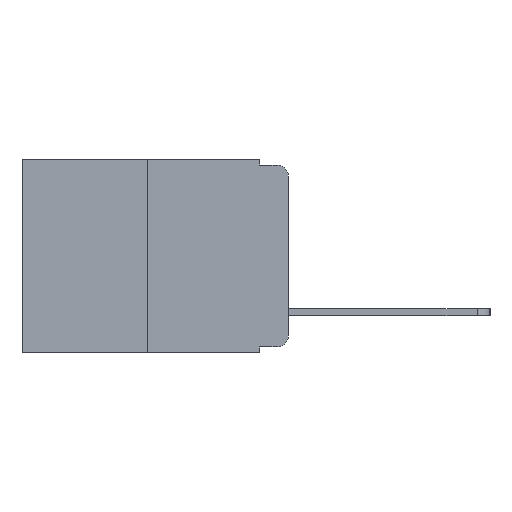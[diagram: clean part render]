
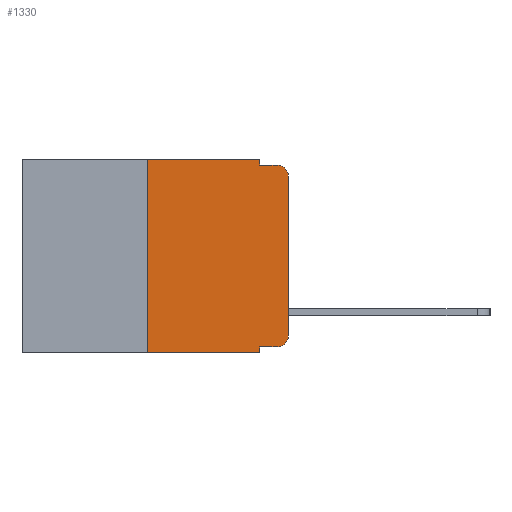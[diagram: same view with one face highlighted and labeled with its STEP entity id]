
A CAD part, left-side view. The second image highlights one B-rep face of the part: STEP entity #1330.
In plain terms, the highlighted planar face has unit normal (-1, 0, 0).
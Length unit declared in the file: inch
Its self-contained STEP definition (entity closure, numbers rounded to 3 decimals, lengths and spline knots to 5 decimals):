
#239 = CARTESIAN_POINT ( 'NONE',  ( 0., 0.473, 0. ) ) ;
#452 = CARTESIAN_POINT ( 'NONE',  ( 0., 0.25, 0. ) ) ;
#518 = DIRECTION ( 'NONE',  ( 0., -1., 0. ) ) ;
#803 = DIRECTION ( 'NONE',  ( 0., 0., 1. ) ) ;
#1142 = CARTESIAN_POINT ( 'NONE',  ( 0., 0.051, -0.01 ) ) ;
#1220 = VERTEX_POINT ( 'NONE', #11399 ) ;
#1290 = LINE ( 'NONE', #6276, #6802 ) ;
#1330 = ADVANCED_FACE ( 'NONE', ( #11483 ), #2594, .F. ) ;
#1460 = LINE ( 'NONE', #11569, #6978 ) ;
#1478 = DIRECTION ( 'NONE',  ( 0., 0., -1. ) ) ;
#1494 = DIRECTION ( 'NONE',  ( 0., -1., 0. ) ) ;
#1685 = DIRECTION ( 'NONE',  ( 0., 0., 1. ) ) ;
#1950 = DIRECTION ( 'NONE',  ( 0., 0., -1. ) ) ;
#2337 = CARTESIAN_POINT ( 'NONE',  ( 0., 0.051, 0. ) ) ;
#2455 = DIRECTION ( 'NONE',  ( 0., 0., -1. ) ) ;
#2460 = VERTEX_POINT ( 'NONE', #4876 ) ;
#2469 = DIRECTION ( 'NONE',  ( 1., 0., 0. ) ) ;
#2594 = PLANE ( 'NONE',  #12680 ) ;
#2900 = CARTESIAN_POINT ( 'NONE',  ( 0., 0.051, -0.01 ) ) ;
#2951 = CIRCLE ( 'NONE', #4506, 0.02 ) ;
#3138 = LINE ( 'NONE', #9721, #13435 ) ;
#3507 = CARTESIAN_POINT ( 'NONE',  ( 0., 0.02, -0.03 ) ) ;
#3771 = VERTEX_POINT ( 'NONE', #1142 ) ;
#4267 = CARTESIAN_POINT ( 'NONE',  ( 0., 0.02, -0.01 ) ) ;
#4317 = LINE ( 'NONE', #452, #6787 ) ;
#4451 = CARTESIAN_POINT ( 'NONE',  ( 0., 0., -0.03 ) ) ;
#4480 = LINE ( 'NONE', #13424, #9572 ) ;
#4506 = AXIS2_PLACEMENT_3D ( 'NONE', #11437, #5471, #12399 ) ;
#4597 = DIRECTION ( 'NONE',  ( 0., 0., -1. ) ) ;
#4876 = CARTESIAN_POINT ( 'NONE',  ( 0., 0.02, -0.333 ) ) ;
#5471 = DIRECTION ( 'NONE',  ( -1., 0., 0. ) ) ;
#5901 = CARTESIAN_POINT ( 'NONE',  ( 0., 0.25, -0.343 ) ) ;
#6015 = EDGE_LOOP ( 'NONE', ( #7263, #7251, #7418, #7274, #7289, #7098, #7149, #6641, #9704, #9143 ) ) ;
#6092 = VERTEX_POINT ( 'NONE', #10795 ) ;
#6276 = CARTESIAN_POINT ( 'NONE',  ( 0., 0., 0. ) ) ;
#6279 = EDGE_CURVE ( 'NONE', #3771, #13244, #11553, .T. ) ;
#6436 = EDGE_CURVE ( 'NONE', #8540, #11033, #1290, .T. ) ;
#6577 = EDGE_CURVE ( 'NONE', #2460, #8540, #2951, .T. ) ;
#6641 = ORIENTED_EDGE ( 'NONE', *, *, #6742, .F. ) ;
#6650 = EDGE_CURVE ( 'NONE', #1220, #2460, #1460, .T. ) ;
#6742 = EDGE_CURVE ( 'NONE', #1220, #9616, #3138, .T. ) ;
#6758 = LINE ( 'NONE', #239, #11659 ) ;
#6787 = VECTOR ( 'NONE', #1685, 39.37008 ) ;
#6802 = VECTOR ( 'NONE', #803, 39.37008 ) ;
#6820 = EDGE_CURVE ( 'NONE', #8948, #6092, #4317, .T. ) ;
#6922 = EDGE_CURVE ( 'NONE', #7778, #3771, #12991, .T. ) ;
#6978 = VECTOR ( 'NONE', #9624, 39.37008 ) ;
#7089 = EDGE_CURVE ( 'NONE', #11033, #13244, #10361, .T. ) ;
#7098 = ORIENTED_EDGE ( 'NONE', *, *, #6820, .F. ) ;
#7119 = CARTESIAN_POINT ( 'NONE',  ( 0., 0.473, 0. ) ) ;
#7149 = ORIENTED_EDGE ( 'NONE', *, *, #7755, .T. ) ;
#7251 = ORIENTED_EDGE ( 'NONE', *, *, #7089, .T. ) ;
#7263 = ORIENTED_EDGE ( 'NONE', *, *, #6436, .T. ) ;
#7274 = ORIENTED_EDGE ( 'NONE', *, *, #6922, .F. ) ;
#7289 = ORIENTED_EDGE ( 'NONE', *, *, #11413, .F. ) ;
#7379 = CARTESIAN_POINT ( 'NONE',  ( 0., 0.051, 0. ) ) ;
#7418 = ORIENTED_EDGE ( 'NONE', *, *, #6279, .F. ) ;
#7726 = DIRECTION ( 'NONE',  ( 0., -1., 0. ) ) ;
#7755 = EDGE_CURVE ( 'NONE', #8948, #9616, #4480, .T. ) ;
#7778 = VERTEX_POINT ( 'NONE', #2337 ) ;
#8540 = VERTEX_POINT ( 'NONE', #9503 ) ;
#8948 = VERTEX_POINT ( 'NONE', #5901 ) ;
#8975 = VECTOR ( 'NONE', #518, 39.37008 ) ;
#9143 = ORIENTED_EDGE ( 'NONE', *, *, #6577, .T. ) ;
#9503 = CARTESIAN_POINT ( 'NONE',  ( 0., 0., -0.313 ) ) ;
#9572 = VECTOR ( 'NONE', #7726, 39.37008 ) ;
#9616 = VERTEX_POINT ( 'NONE', #9665 ) ;
#9624 = DIRECTION ( 'NONE',  ( 0., -1., 0. ) ) ;
#9665 = CARTESIAN_POINT ( 'NONE',  ( 0., 0.051, -0.343 ) ) ;
#9704 = ORIENTED_EDGE ( 'NONE', *, *, #6650, .T. ) ;
#9721 = CARTESIAN_POINT ( 'NONE',  ( 0., 0.051, 0. ) ) ;
#10219 = VECTOR ( 'NONE', #1950, 39.37008 ) ;
#10361 = CIRCLE ( 'NONE', #11649, 0.02 ) ;
#10653 = DIRECTION ( 'NONE',  ( -1., 0., 0. ) ) ;
#10795 = CARTESIAN_POINT ( 'NONE',  ( 0., 0.25, 0. ) ) ;
#11033 = VERTEX_POINT ( 'NONE', #4451 ) ;
#11399 = CARTESIAN_POINT ( 'NONE',  ( 0., 0.051, -0.333 ) ) ;
#11413 = EDGE_CURVE ( 'NONE', #6092, #7778, #6758, .T. ) ;
#11437 = CARTESIAN_POINT ( 'NONE',  ( 0., 0.02, -0.313 ) ) ;
#11483 = FACE_OUTER_BOUND ( 'NONE', #6015, .T. ) ;
#11553 = LINE ( 'NONE', #2900, #8975 ) ;
#11569 = CARTESIAN_POINT ( 'NONE',  ( 0., 0.051, -0.333 ) ) ;
#11649 = AXIS2_PLACEMENT_3D ( 'NONE', #3507, #10653, #4597 ) ;
#11659 = VECTOR ( 'NONE', #1494, 39.37008 ) ;
#12399 = DIRECTION ( 'NONE',  ( 0., 0., -1. ) ) ;
#12680 = AXIS2_PLACEMENT_3D ( 'NONE', #7119, #2469, #2455 ) ;
#12991 = LINE ( 'NONE', #7379, #10219 ) ;
#13244 = VERTEX_POINT ( 'NONE', #4267 ) ;
#13424 = CARTESIAN_POINT ( 'NONE',  ( 0., 0.473, -0.343 ) ) ;
#13435 = VECTOR ( 'NONE', #1478, 39.37008 ) ;
